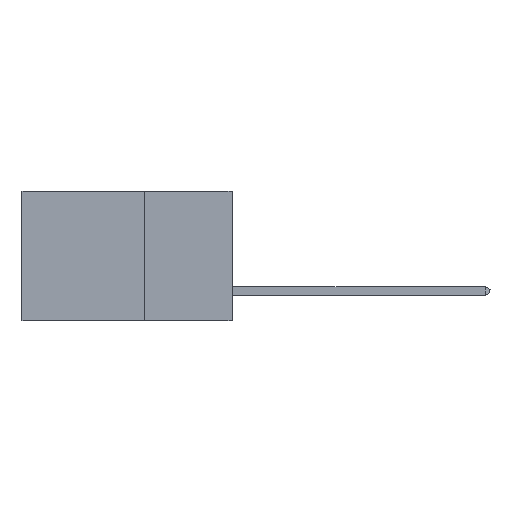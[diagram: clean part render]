
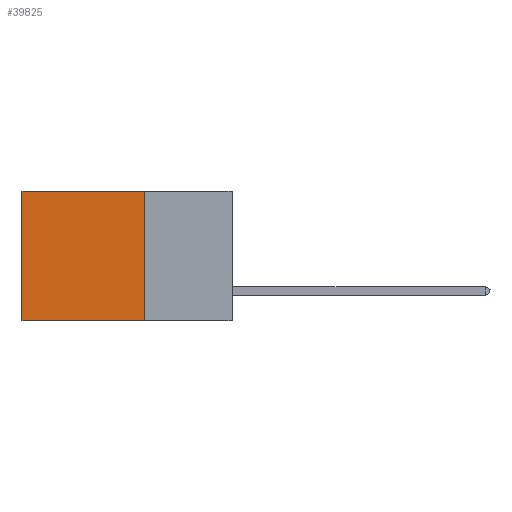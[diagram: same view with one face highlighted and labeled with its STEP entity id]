
A CAD part, left-side view. The second image highlights one B-rep face of the part: STEP entity #39825.
In plain terms, the highlighted planar face has unit normal (-1, 0, 0).
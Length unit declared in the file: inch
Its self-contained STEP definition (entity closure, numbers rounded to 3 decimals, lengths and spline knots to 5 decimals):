
#750 = FACE_OUTER_BOUND ( 'NONE', #21601, .T. ) ;
#2454 = DIRECTION ( 'NONE',  ( 0., 1., 0. ) ) ;
#2540 = VERTEX_POINT ( 'NONE', #3685 ) ;
#3685 = CARTESIAN_POINT ( 'NONE',  ( 0.2875, 0.6, 0. ) ) ;
#3857 = VECTOR ( 'NONE', #2454, 39.37008 ) ;
#4771 = DIRECTION ( 'NONE',  ( 1., 0., 0. ) ) ;
#5155 = VECTOR ( 'NONE', #10789, 39.37008 ) ;
#5361 = LINE ( 'NONE', #10277, #41208 ) ;
#8558 = DIRECTION ( 'NONE',  ( 0., 0., -1. ) ) ;
#10277 = CARTESIAN_POINT ( 'NONE',  ( 0.2875, 0.25, 0. ) ) ;
#10789 = DIRECTION ( 'NONE',  ( 0., 1., 0. ) ) ;
#11232 = AXIS2_PLACEMENT_3D ( 'NONE', #11602, #4771, #8558 ) ;
#11602 = CARTESIAN_POINT ( 'NONE',  ( 0.2875, 0.25, 0. ) ) ;
#13092 = LINE ( 'NONE', #33560, #3857 ) ;
#13927 = EDGE_CURVE ( 'NONE', #37585, #44694, #5361, .T. ) ;
#14025 = CARTESIAN_POINT ( 'NONE',  ( 0.2875, 0.25, -0.37 ) ) ;
#16390 = CARTESIAN_POINT ( 'NONE',  ( 0.2875, 0.25, 0. ) ) ;
#17964 = DIRECTION ( 'NONE',  ( 0., 0., -1. ) ) ;
#19893 = CARTESIAN_POINT ( 'NONE',  ( 0.2875, 0.6, 0. ) ) ;
#21601 = EDGE_LOOP ( 'NONE', ( #29153, #41293, #44873, #23008 ) ) ;
#23008 = ORIENTED_EDGE ( 'NONE', *, *, #37745, .T. ) ;
#24588 = CARTESIAN_POINT ( 'NONE',  ( 0.2875, 0.25, 0. ) ) ;
#26131 = LINE ( 'NONE', #19893, #30539 ) ;
#26277 = LINE ( 'NONE', #24588, #5155 ) ;
#26736 = CARTESIAN_POINT ( 'NONE',  ( 0.2875, 0.6, -0.37 ) ) ;
#29153 = ORIENTED_EDGE ( 'NONE', *, *, #33490, .T. ) ;
#30539 = VECTOR ( 'NONE', #44264, 39.37008 ) ;
#33490 = EDGE_CURVE ( 'NONE', #2540, #40023, #26131, .T. ) ;
#33560 = CARTESIAN_POINT ( 'NONE',  ( 0.2875, 0.25, -0.37 ) ) ;
#33935 = EDGE_CURVE ( 'NONE', #44694, #40023, #13092, .T. ) ;
#36164 = PLANE ( 'NONE',  #11232 ) ;
#37585 = VERTEX_POINT ( 'NONE', #16390 ) ;
#37745 = EDGE_CURVE ( 'NONE', #37585, #2540, #26277, .T. ) ;
#39825 = ADVANCED_FACE ( 'NONE', ( #750 ), #36164, .F. ) ;
#40023 = VERTEX_POINT ( 'NONE', #26736 ) ;
#41208 = VECTOR ( 'NONE', #17964, 39.37008 ) ;
#41293 = ORIENTED_EDGE ( 'NONE', *, *, #33935, .F. ) ;
#44264 = DIRECTION ( 'NONE',  ( 0., 0., -1. ) ) ;
#44694 = VERTEX_POINT ( 'NONE', #14025 ) ;
#44873 = ORIENTED_EDGE ( 'NONE', *, *, #13927, .F. ) ;
